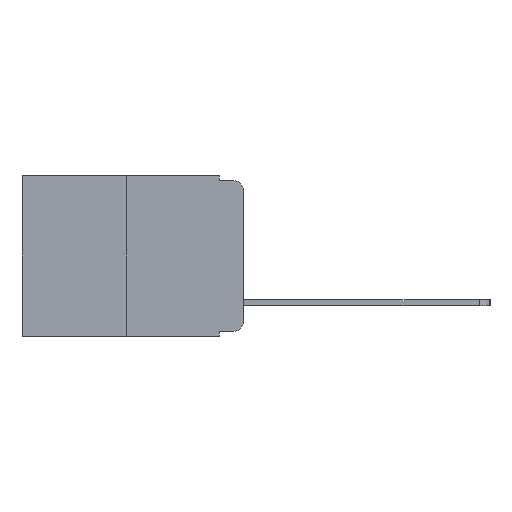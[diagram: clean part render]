
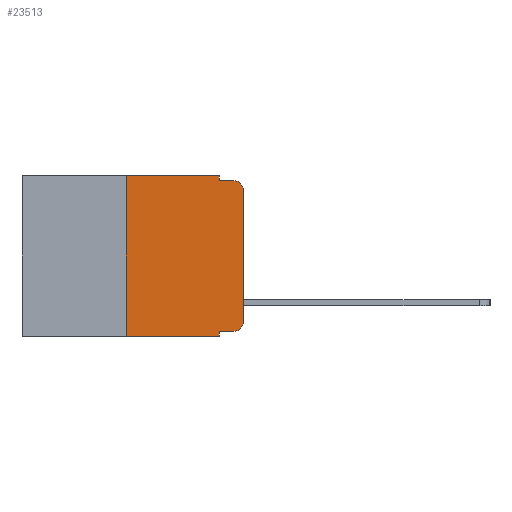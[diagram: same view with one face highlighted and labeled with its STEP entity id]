
A CAD part, left-side view. The second image highlights one B-rep face of the part: STEP entity #23513.
In plain terms, the highlighted planar face has unit normal (-1, 0, 0).
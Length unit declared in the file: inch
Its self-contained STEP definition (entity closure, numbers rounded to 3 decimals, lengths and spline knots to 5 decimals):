
#74 = ORIENTED_EDGE ( 'NONE', *, *, #14689, .F. ) ;
#264 = VECTOR ( 'NONE', #13878, 39.37008 ) ;
#567 = EDGE_CURVE ( 'NONE', #20310, #6273, #15584, .T. ) ;
#679 = DIRECTION ( 'NONE',  ( -1., 0., 0. ) ) ;
#739 = CARTESIAN_POINT ( 'NONE',  ( 0., 0.051, -0.343 ) ) ;
#1333 = ORIENTED_EDGE ( 'NONE', *, *, #14238, .F. ) ;
#1560 = VECTOR ( 'NONE', #21682, 39.37008 ) ;
#2126 = CARTESIAN_POINT ( 'NONE',  ( 0., 0.02, -0.313 ) ) ;
#2616 = ORIENTED_EDGE ( 'NONE', *, *, #5077, .F. ) ;
#3535 = AXIS2_PLACEMENT_3D ( 'NONE', #12778, #679, #14674 ) ;
#3570 = ORIENTED_EDGE ( 'NONE', *, *, #3666, .T. ) ;
#3666 = EDGE_CURVE ( 'NONE', #12658, #23253, #8012, .T. ) ;
#3926 = ORIENTED_EDGE ( 'NONE', *, *, #567, .T. ) ;
#4188 = DIRECTION ( 'NONE',  ( 0., 0., -1. ) ) ;
#4357 = VERTEX_POINT ( 'NONE', #7450 ) ;
#5012 = CARTESIAN_POINT ( 'NONE',  ( 0., 0.02, -0.333 ) ) ;
#5077 = EDGE_CURVE ( 'NONE', #20310, #9358, #7324, .T. ) ;
#5712 = AXIS2_PLACEMENT_3D ( 'NONE', #2126, #16016, #4188 ) ;
#6273 = VERTEX_POINT ( 'NONE', #5012 ) ;
#6671 = EDGE_CURVE ( 'NONE', #23253, #13149, #21343, .T. ) ;
#6701 = CARTESIAN_POINT ( 'NONE',  ( 0., 0.051, -0.333 ) ) ;
#6728 = ORIENTED_EDGE ( 'NONE', *, *, #17588, .F. ) ;
#6794 = DIRECTION ( 'NONE',  ( 0., -1., 0. ) ) ;
#7324 = LINE ( 'NONE', #17238, #11434 ) ;
#7450 = CARTESIAN_POINT ( 'NONE',  ( 0., 0.25, -0.343 ) ) ;
#8012 = LINE ( 'NONE', #13896, #22696 ) ;
#9358 = VERTEX_POINT ( 'NONE', #739 ) ;
#9674 = VECTOR ( 'NONE', #22872, 39.37008 ) ;
#10027 = VECTOR ( 'NONE', #20237, 39.37008 ) ;
#10031 = EDGE_LOOP ( 'NONE', ( #3570, #20331, #74, #10816, #1333, #6728, #17746, #2616, #3926, #20064 ) ) ;
#10076 = CARTESIAN_POINT ( 'NONE',  ( 0., 0.473, 0. ) ) ;
#10646 = LINE ( 'NONE', #20077, #10027 ) ;
#10816 = ORIENTED_EDGE ( 'NONE', *, *, #23099, .F. ) ;
#11079 = CARTESIAN_POINT ( 'NONE',  ( 0., 0.051, 0. ) ) ;
#11211 = LINE ( 'NONE', #12571, #16343 ) ;
#11434 = VECTOR ( 'NONE', #19130, 39.37008 ) ;
#11726 = CARTESIAN_POINT ( 'NONE',  ( 0., 0.051, -0.01 ) ) ;
#12080 = DIRECTION ( 'NONE',  ( 0., 0., -1. ) ) ;
#12571 = CARTESIAN_POINT ( 'NONE',  ( 0., 0.25, 0. ) ) ;
#12658 = VERTEX_POINT ( 'NONE', #22890 ) ;
#12778 = CARTESIAN_POINT ( 'NONE',  ( 0., 0.02, -0.03 ) ) ;
#12907 = LINE ( 'NONE', #19834, #1560 ) ;
#13149 = VERTEX_POINT ( 'NONE', #22555 ) ;
#13244 = CARTESIAN_POINT ( 'NONE',  ( 0., 0., -0.03 ) ) ;
#13497 = CARTESIAN_POINT ( 'NONE',  ( 0., 0.473, -0.343 ) ) ;
#13571 = DIRECTION ( 'NONE',  ( 0., 0., 1. ) ) ;
#13878 = DIRECTION ( 'NONE',  ( 0., -1., 0. ) ) ;
#13896 = CARTESIAN_POINT ( 'NONE',  ( 0., 0., 0. ) ) ;
#14238 = EDGE_CURVE ( 'NONE', #16625, #17743, #12907, .T. ) ;
#14287 = CARTESIAN_POINT ( 'NONE',  ( 0., 0.051, -0.333 ) ) ;
#14674 = DIRECTION ( 'NONE',  ( 0., 0., -1. ) ) ;
#14689 = EDGE_CURVE ( 'NONE', #22784, #13149, #15544, .T. ) ;
#14967 = VECTOR ( 'NONE', #6794, 39.37008 ) ;
#15413 = EDGE_CURVE ( 'NONE', #6273, #12658, #25127, .T. ) ;
#15481 = LINE ( 'NONE', #13497, #9674 ) ;
#15544 = LINE ( 'NONE', #25071, #264 ) ;
#15584 = LINE ( 'NONE', #6701, #14967 ) ;
#16016 = DIRECTION ( 'NONE',  ( -1., 0., 0. ) ) ;
#16343 = VECTOR ( 'NONE', #23791, 39.37008 ) ;
#16625 = VERTEX_POINT ( 'NONE', #18915 ) ;
#17238 = CARTESIAN_POINT ( 'NONE',  ( 0., 0.051, 0. ) ) ;
#17588 = EDGE_CURVE ( 'NONE', #4357, #16625, #11211, .T. ) ;
#17743 = VERTEX_POINT ( 'NONE', #11079 ) ;
#17746 = ORIENTED_EDGE ( 'NONE', *, *, #23349, .T. ) ;
#18915 = CARTESIAN_POINT ( 'NONE',  ( 0., 0.25, 0. ) ) ;
#19130 = DIRECTION ( 'NONE',  ( 0., 0., -1. ) ) ;
#19834 = CARTESIAN_POINT ( 'NONE',  ( 0., 0.473, 0. ) ) ;
#20064 = ORIENTED_EDGE ( 'NONE', *, *, #15413, .T. ) ;
#20077 = CARTESIAN_POINT ( 'NONE',  ( 0., 0.051, 0. ) ) ;
#20237 = DIRECTION ( 'NONE',  ( 0., 0., -1. ) ) ;
#20310 = VERTEX_POINT ( 'NONE', #14287 ) ;
#20331 = ORIENTED_EDGE ( 'NONE', *, *, #6671, .T. ) ;
#20733 = FACE_OUTER_BOUND ( 'NONE', #10031, .T. ) ;
#21343 = CIRCLE ( 'NONE', #3535, 0.02 ) ;
#21459 = PLANE ( 'NONE',  #23082 ) ;
#21682 = DIRECTION ( 'NONE',  ( 0., -1., 0. ) ) ;
#22555 = CARTESIAN_POINT ( 'NONE',  ( 0., 0.02, -0.01 ) ) ;
#22696 = VECTOR ( 'NONE', #13571, 39.37008 ) ;
#22784 = VERTEX_POINT ( 'NONE', #11726 ) ;
#22872 = DIRECTION ( 'NONE',  ( 0., -1., 0. ) ) ;
#22890 = CARTESIAN_POINT ( 'NONE',  ( 0., 0., -0.313 ) ) ;
#23082 = AXIS2_PLACEMENT_3D ( 'NONE', #10076, #23322, #12080 ) ;
#23099 = EDGE_CURVE ( 'NONE', #17743, #22784, #10646, .T. ) ;
#23253 = VERTEX_POINT ( 'NONE', #13244 ) ;
#23322 = DIRECTION ( 'NONE',  ( 1., 0., 0. ) ) ;
#23349 = EDGE_CURVE ( 'NONE', #4357, #9358, #15481, .T. ) ;
#23513 = ADVANCED_FACE ( 'NONE', ( #20733 ), #21459, .F. ) ;
#23791 = DIRECTION ( 'NONE',  ( 0., 0., 1. ) ) ;
#25071 = CARTESIAN_POINT ( 'NONE',  ( 0., 0.051, -0.01 ) ) ;
#25127 = CIRCLE ( 'NONE', #5712, 0.02 ) ;
